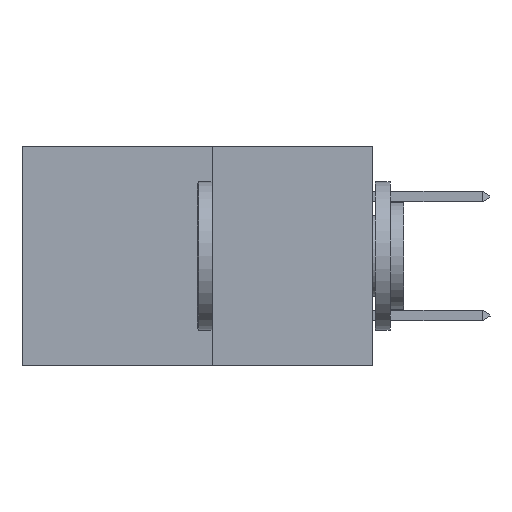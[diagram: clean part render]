
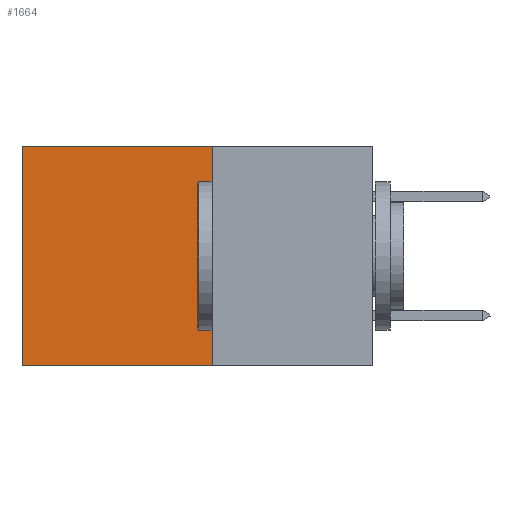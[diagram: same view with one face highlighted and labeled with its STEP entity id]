
A CAD part, left-side view. The second image highlights one B-rep face of the part: STEP entity #1664.
In plain terms, the highlighted planar face has unit normal (-1, 0, 0).
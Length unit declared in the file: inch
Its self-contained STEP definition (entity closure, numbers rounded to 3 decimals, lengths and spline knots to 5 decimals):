
#54 = EDGE_CURVE ( 'NONE', #5242, #8873, #1702, .T. ) ;
#294 = VECTOR ( 'NONE', #7212, 39.37008 ) ;
#1115 = LINE ( 'NONE', #2856, #4935 ) ;
#1303 = AXIS2_PLACEMENT_3D ( 'NONE', #9706, #2954, #7591 ) ;
#1664 = ADVANCED_FACE ( 'NONE', ( #2350 ), #4245, .F. ) ;
#1702 = LINE ( 'NONE', #2011, #7635 ) ;
#2011 = CARTESIAN_POINT ( 'NONE',  ( 0.277, 0.59, -0.37 ) ) ;
#2071 = EDGE_CURVE ( 'NONE', #2764, #5242, #4417, .T. ) ;
#2350 = FACE_OUTER_BOUND ( 'NONE', #7019, .T. ) ;
#2695 = EDGE_CURVE ( 'NONE', #2764, #9386, #2964, .T. ) ;
#2746 = CARTESIAN_POINT ( 'NONE',  ( 0.277, 0.27, -0.37 ) ) ;
#2764 = VERTEX_POINT ( 'NONE', #6586 ) ;
#2856 = CARTESIAN_POINT ( 'NONE',  ( 0.277, 0.27, -0.37 ) ) ;
#2954 = DIRECTION ( 'NONE',  ( 1., 0., 0. ) ) ;
#2964 = LINE ( 'NONE', #7142, #294 ) ;
#3362 = DIRECTION ( 'NONE',  ( 0., 1., 0. ) ) ;
#3408 = CARTESIAN_POINT ( 'NONE',  ( 0.277, 0.27, 0. ) ) ;
#3922 = DIRECTION ( 'NONE',  ( 0., 0., -1. ) ) ;
#3953 = ORIENTED_EDGE ( 'NONE', *, *, #9584, .F. ) ;
#4245 = PLANE ( 'NONE',  #1303 ) ;
#4417 = LINE ( 'NONE', #3408, #7109 ) ;
#4426 = DIRECTION ( 'NONE',  ( 0., 1., 0. ) ) ;
#4709 = ORIENTED_EDGE ( 'NONE', *, *, #2071, .T. ) ;
#4758 = ORIENTED_EDGE ( 'NONE', *, *, #54, .T. ) ;
#4935 = VECTOR ( 'NONE', #4426, 39.37008 ) ;
#5242 = VERTEX_POINT ( 'NONE', #9847 ) ;
#5786 = ORIENTED_EDGE ( 'NONE', *, *, #2695, .F. ) ;
#6586 = CARTESIAN_POINT ( 'NONE',  ( 0.277, 0.27, 0. ) ) ;
#7019 = EDGE_LOOP ( 'NONE', ( #4758, #3953, #5786, #4709 ) ) ;
#7109 = VECTOR ( 'NONE', #3362, 39.37008 ) ;
#7142 = CARTESIAN_POINT ( 'NONE',  ( 0.277, 0.27, -0.37 ) ) ;
#7212 = DIRECTION ( 'NONE',  ( 0., 0., -1. ) ) ;
#7591 = DIRECTION ( 'NONE',  ( 0., 0., -1. ) ) ;
#7635 = VECTOR ( 'NONE', #3922, 39.37008 ) ;
#7655 = CARTESIAN_POINT ( 'NONE',  ( 0.277, 0.59, -0.37 ) ) ;
#8873 = VERTEX_POINT ( 'NONE', #7655 ) ;
#9386 = VERTEX_POINT ( 'NONE', #2746 ) ;
#9584 = EDGE_CURVE ( 'NONE', #9386, #8873, #1115, .T. ) ;
#9706 = CARTESIAN_POINT ( 'NONE',  ( 0.277, 0.27, -0.37 ) ) ;
#9847 = CARTESIAN_POINT ( 'NONE',  ( 0.277, 0.59, 0. ) ) ;
